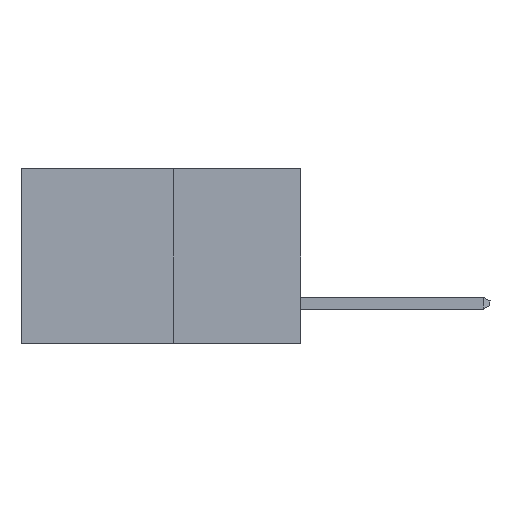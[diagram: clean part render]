
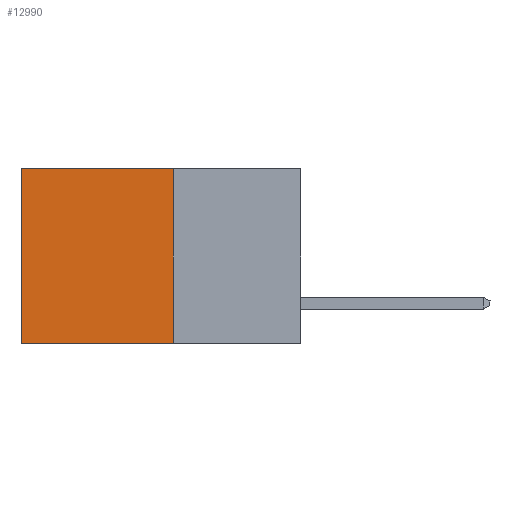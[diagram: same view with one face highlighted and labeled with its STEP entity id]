
A CAD part, left-side view. The second image highlights one B-rep face of the part: STEP entity #12990.
In plain terms, the highlighted planar face has unit normal (-1, 0, 0).
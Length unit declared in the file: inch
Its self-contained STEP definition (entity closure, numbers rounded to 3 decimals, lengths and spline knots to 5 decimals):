
#115 = CARTESIAN_POINT ( 'NONE',  ( 0.277, 0.27, 0. ) ) ;
#323 = DIRECTION ( 'NONE',  ( 0., 1., 0. ) ) ;
#324 = VERTEX_POINT ( 'NONE', #10350 ) ;
#715 = ORIENTED_EDGE ( 'NONE', *, *, #4910, .T. ) ;
#1052 = PLANE ( 'NONE',  #3453 ) ;
#1627 = LINE ( 'NONE', #4205, #9845 ) ;
#1803 = LINE ( 'NONE', #115, #4905 ) ;
#1811 = CARTESIAN_POINT ( 'NONE',  ( 0.277, 0.59, -0.37 ) ) ;
#1890 = DIRECTION ( 'NONE',  ( 0., 0., -1. ) ) ;
#2030 = EDGE_CURVE ( 'NONE', #14097, #12243, #3019, .T. ) ;
#2312 = CARTESIAN_POINT ( 'NONE',  ( 0.277, 0.27, -0.37 ) ) ;
#3019 = LINE ( 'NONE', #13722, #14039 ) ;
#3227 = ORIENTED_EDGE ( 'NONE', *, *, #6873, .T. ) ;
#3453 = AXIS2_PLACEMENT_3D ( 'NONE', #2312, #10069, #3501 ) ;
#3501 = DIRECTION ( 'NONE',  ( 0., 0., -1. ) ) ;
#3592 = ORIENTED_EDGE ( 'NONE', *, *, #6708, .F. ) ;
#3598 = CARTESIAN_POINT ( 'NONE',  ( 0.277, 0.59, 0. ) ) ;
#4205 = CARTESIAN_POINT ( 'NONE',  ( 0.277, 0.27, -0.37 ) ) ;
#4381 = DIRECTION ( 'NONE',  ( 0., 0., -1. ) ) ;
#4619 = EDGE_LOOP ( 'NONE', ( #3227, #12006, #3592, #715 ) ) ;
#4905 = VECTOR ( 'NONE', #323, 39.37008 ) ;
#4910 = EDGE_CURVE ( 'NONE', #324, #8818, #1803, .T. ) ;
#6367 = CARTESIAN_POINT ( 'NONE',  ( 0.277, 0.59, -0.37 ) ) ;
#6708 = EDGE_CURVE ( 'NONE', #324, #14097, #1627, .T. ) ;
#6873 = EDGE_CURVE ( 'NONE', #8818, #12243, #13636, .T. ) ;
#8818 = VERTEX_POINT ( 'NONE', #3598 ) ;
#9714 = FACE_OUTER_BOUND ( 'NONE', #4619, .T. ) ;
#9845 = VECTOR ( 'NONE', #4381, 39.37008 ) ;
#10069 = DIRECTION ( 'NONE',  ( 1., 0., 0. ) ) ;
#10350 = CARTESIAN_POINT ( 'NONE',  ( 0.277, 0.27, 0. ) ) ;
#10370 = VECTOR ( 'NONE', #1890, 39.37008 ) ;
#11014 = CARTESIAN_POINT ( 'NONE',  ( 0.277, 0.27, -0.37 ) ) ;
#12006 = ORIENTED_EDGE ( 'NONE', *, *, #2030, .F. ) ;
#12243 = VERTEX_POINT ( 'NONE', #6367 ) ;
#12615 = DIRECTION ( 'NONE',  ( 0., 1., 0. ) ) ;
#12990 = ADVANCED_FACE ( 'NONE', ( #9714 ), #1052, .F. ) ;
#13636 = LINE ( 'NONE', #1811, #10370 ) ;
#13722 = CARTESIAN_POINT ( 'NONE',  ( 0.277, 0.27, -0.37 ) ) ;
#14039 = VECTOR ( 'NONE', #12615, 39.37008 ) ;
#14097 = VERTEX_POINT ( 'NONE', #11014 ) ;
